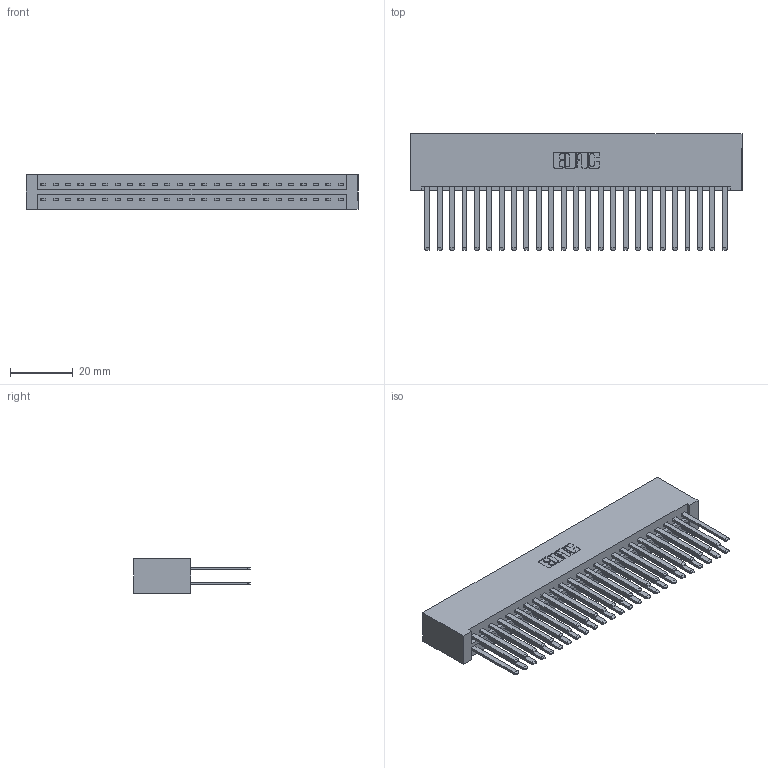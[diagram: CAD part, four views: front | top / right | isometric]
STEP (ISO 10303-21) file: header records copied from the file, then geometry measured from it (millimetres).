
FILE_DESCRIPTION (( 'STEP AP203' ), '1' );
FILE_NAME ('336-050-541-801.STEP', '2020-08-08T00:06:50', ( '' ), ( '' ), 'SwSTEP 2.0', 'SolidWorks 2020', '' );
FILE_SCHEMA (( 'CONFIG_CONTROL_DESIGN' ));
Length unit declared in the file: inch
Products named in the file (3): 336-050-541-801; 336 Part_Lugless; 336-290-001_336-290-541
Assembly tree (51 placements, depth 2):
  336-050-541-801
    336 Part_Lugless
    336-290-001_336-290-541  x50
Bounding box: 106.17 x 37.34 x 11.1 mm (x, y, z)
Volume: 17527.6 mm3; surface area: 22269 mm2
Topology: 51 solids, 51 shells, 2206 faces, 6637 edges, 4390 vertices
Faces by surface type: plane 1366, cylinder 840
Entity records: 21024 total; most frequent: CARTESIAN_POINT 3637, ORIENTED_EDGE 3474, DIRECTION 3021, EDGE_CURVE 1737, LINE 1613, VECTOR 1613, VERTEX_POINT 1156, AXIS2_PLACEMENT_3D 704
